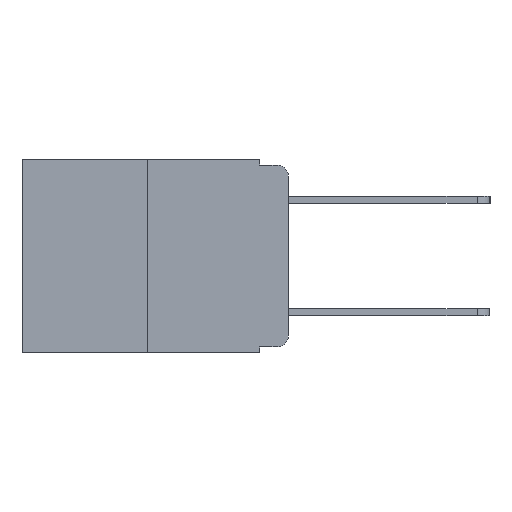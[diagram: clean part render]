
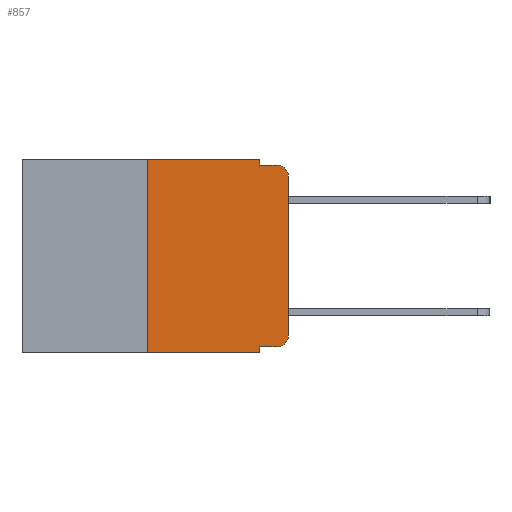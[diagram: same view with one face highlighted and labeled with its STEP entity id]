
A CAD part, left-side view. The second image highlights one B-rep face of the part: STEP entity #857.
In plain terms, the highlighted planar face has unit normal (-1, 0, 0).
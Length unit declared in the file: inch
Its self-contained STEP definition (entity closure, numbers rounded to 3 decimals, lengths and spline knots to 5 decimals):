
#37 = VECTOR ( 'NONE', #664, 39.37008 ) ;
#220 = ORIENTED_EDGE ( 'NONE', *, *, #5882, .T. ) ;
#239 = LINE ( 'NONE', #734, #3440 ) ;
#391 = DIRECTION ( 'NONE',  ( 0., 0., 1. ) ) ;
#552 = VECTOR ( 'NONE', #14397, 39.37008 ) ;
#664 = DIRECTION ( 'NONE',  ( 0., 0., -1. ) ) ;
#671 = DIRECTION ( 'NONE',  ( 0., -1., 0. ) ) ;
#734 = CARTESIAN_POINT ( 'NONE',  ( 0., 0.473, -0.343 ) ) ;
#857 = ADVANCED_FACE ( 'NONE', ( #8877 ), #2823, .F. ) ;
#2030 = CARTESIAN_POINT ( 'NONE',  ( 0., 0.051, -0.01 ) ) ;
#2062 = CARTESIAN_POINT ( 'NONE',  ( 0., 0.051, 0. ) ) ;
#2278 = LINE ( 'NONE', #5670, #9395 ) ;
#2280 = CARTESIAN_POINT ( 'NONE',  ( 0., 0.051, -0.333 ) ) ;
#2383 = VERTEX_POINT ( 'NONE', #12730 ) ;
#2499 = DIRECTION ( 'NONE',  ( -1., 0., 0. ) ) ;
#2782 = VERTEX_POINT ( 'NONE', #10529 ) ;
#2823 = PLANE ( 'NONE',  #7105 ) ;
#2835 = VERTEX_POINT ( 'NONE', #5776 ) ;
#2843 = AXIS2_PLACEMENT_3D ( 'NONE', #11923, #4397, #13159 ) ;
#3440 = VECTOR ( 'NONE', #9699, 39.37008 ) ;
#3729 = ORIENTED_EDGE ( 'NONE', *, *, #11094, .T. ) ;
#4077 = LINE ( 'NONE', #13267, #552 ) ;
#4310 = ORIENTED_EDGE ( 'NONE', *, *, #12149, .T. ) ;
#4397 = DIRECTION ( 'NONE',  ( -1., 0., 0. ) ) ;
#4486 = ORIENTED_EDGE ( 'NONE', *, *, #11328, .F. ) ;
#4569 = CARTESIAN_POINT ( 'NONE',  ( 0., 0.473, 0. ) ) ;
#4753 = ORIENTED_EDGE ( 'NONE', *, *, #11188, .F. ) ;
#4864 = VERTEX_POINT ( 'NONE', #2030 ) ;
#5132 = CARTESIAN_POINT ( 'NONE',  ( 0., 0.051, -0.343 ) ) ;
#5254 = VECTOR ( 'NONE', #391, 39.37008 ) ;
#5670 = CARTESIAN_POINT ( 'NONE',  ( 0., 0.051, 0. ) ) ;
#5776 = CARTESIAN_POINT ( 'NONE',  ( 0., 0.25, 0. ) ) ;
#5882 = EDGE_CURVE ( 'NONE', #6315, #10379, #239, .T. ) ;
#5896 = ORIENTED_EDGE ( 'NONE', *, *, #11617, .F. ) ;
#6281 = VECTOR ( 'NONE', #13515, 39.37008 ) ;
#6315 = VERTEX_POINT ( 'NONE', #8275 ) ;
#6498 = VERTEX_POINT ( 'NONE', #10008 ) ;
#7105 = AXIS2_PLACEMENT_3D ( 'NONE', #9032, #13810, #7775 ) ;
#7775 = DIRECTION ( 'NONE',  ( 0., 0., -1. ) ) ;
#7981 = CIRCLE ( 'NONE', #12574, 0.02 ) ;
#8033 = ORIENTED_EDGE ( 'NONE', *, *, #11234, .F. ) ;
#8275 = CARTESIAN_POINT ( 'NONE',  ( 0., 0.25, -0.343 ) ) ;
#8471 = VERTEX_POINT ( 'NONE', #11706 ) ;
#8583 = CIRCLE ( 'NONE', #2843, 0.02 ) ;
#8877 = FACE_OUTER_BOUND ( 'NONE', #15950, .T. ) ;
#9032 = CARTESIAN_POINT ( 'NONE',  ( 0., 0.473, 0. ) ) ;
#9176 = LINE ( 'NONE', #2280, #15922 ) ;
#9395 = VECTOR ( 'NONE', #13148, 39.37008 ) ;
#9666 = ORIENTED_EDGE ( 'NONE', *, *, #11096, .T. ) ;
#9699 = DIRECTION ( 'NONE',  ( 0., -1., 0. ) ) ;
#9863 = DIRECTION ( 'NONE',  ( 0., -1., 0. ) ) ;
#10008 = CARTESIAN_POINT ( 'NONE',  ( 0., 0.02, -0.333 ) ) ;
#10064 = CARTESIAN_POINT ( 'NONE',  ( 0., 0.02, -0.313 ) ) ;
#10197 = ORIENTED_EDGE ( 'NONE', *, *, #12073, .T. ) ;
#10379 = VERTEX_POINT ( 'NONE', #5132 ) ;
#10452 = VERTEX_POINT ( 'NONE', #15066 ) ;
#10529 = CARTESIAN_POINT ( 'NONE',  ( 0., 0.02, -0.01 ) ) ;
#11094 = EDGE_CURVE ( 'NONE', #10452, #2383, #15049, .T. ) ;
#11096 = EDGE_CURVE ( 'NONE', #2383, #2782, #8583, .T. ) ;
#11188 = EDGE_CURVE ( 'NONE', #4864, #2782, #4077, .T. ) ;
#11234 = EDGE_CURVE ( 'NONE', #8471, #4864, #13976, .T. ) ;
#11310 = DIRECTION ( 'NONE',  ( 0., 0., -1. ) ) ;
#11328 = EDGE_CURVE ( 'NONE', #6315, #2835, #15226, .T. ) ;
#11617 = EDGE_CURVE ( 'NONE', #12765, #10379, #2278, .T. ) ;
#11706 = CARTESIAN_POINT ( 'NONE',  ( 0., 0.051, 0. ) ) ;
#11869 = CARTESIAN_POINT ( 'NONE',  ( 0., 0., 0. ) ) ;
#11923 = CARTESIAN_POINT ( 'NONE',  ( 0., 0.02, -0.03 ) ) ;
#12073 = EDGE_CURVE ( 'NONE', #12765, #6498, #9176, .T. ) ;
#12149 = EDGE_CURVE ( 'NONE', #6498, #10452, #7981, .T. ) ;
#12305 = CARTESIAN_POINT ( 'NONE',  ( 0., 0.25, 0. ) ) ;
#12574 = AXIS2_PLACEMENT_3D ( 'NONE', #10064, #2499, #11310 ) ;
#12730 = CARTESIAN_POINT ( 'NONE',  ( 0., 0., -0.03 ) ) ;
#12765 = VERTEX_POINT ( 'NONE', #15858 ) ;
#13148 = DIRECTION ( 'NONE',  ( 0., 0., -1. ) ) ;
#13159 = DIRECTION ( 'NONE',  ( 0., 0., -1. ) ) ;
#13267 = CARTESIAN_POINT ( 'NONE',  ( 0., 0.051, -0.01 ) ) ;
#13393 = VECTOR ( 'NONE', #671, 39.37008 ) ;
#13515 = DIRECTION ( 'NONE',  ( 0., 0., 1. ) ) ;
#13661 = ORIENTED_EDGE ( 'NONE', *, *, #15860, .F. ) ;
#13738 = LINE ( 'NONE', #4569, #13393 ) ;
#13810 = DIRECTION ( 'NONE',  ( 1., 0., 0. ) ) ;
#13976 = LINE ( 'NONE', #2062, #37 ) ;
#14397 = DIRECTION ( 'NONE',  ( 0., -1., 0. ) ) ;
#15049 = LINE ( 'NONE', #11869, #5254 ) ;
#15066 = CARTESIAN_POINT ( 'NONE',  ( 0., 0., -0.313 ) ) ;
#15226 = LINE ( 'NONE', #12305, #6281 ) ;
#15858 = CARTESIAN_POINT ( 'NONE',  ( 0., 0.051, -0.333 ) ) ;
#15860 = EDGE_CURVE ( 'NONE', #2835, #8471, #13738, .T. ) ;
#15922 = VECTOR ( 'NONE', #9863, 39.37008 ) ;
#15950 = EDGE_LOOP ( 'NONE', ( #3729, #9666, #4753, #8033, #13661, #4486, #220, #5896, #10197, #4310 ) ) ;
